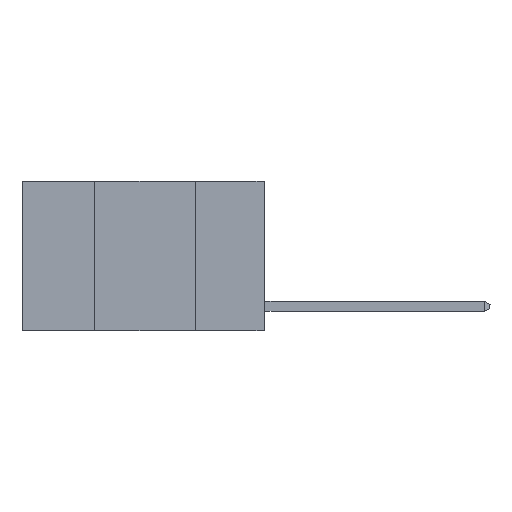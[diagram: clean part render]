
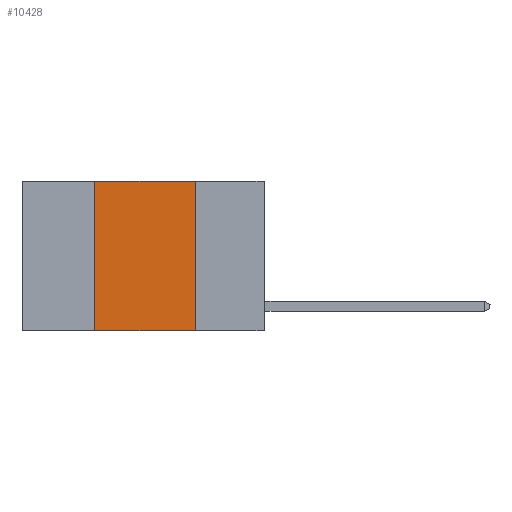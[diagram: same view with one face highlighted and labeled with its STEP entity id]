
A CAD part, left-side view. The second image highlights one B-rep face of the part: STEP entity #10428.
In plain terms, the highlighted planar face has unit normal (-1, 0, 0).
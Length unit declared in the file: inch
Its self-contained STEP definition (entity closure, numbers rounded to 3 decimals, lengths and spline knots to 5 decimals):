
#43 = VERTEX_POINT ( 'NONE', #5023 ) ;
#239 = VECTOR ( 'NONE', #8701, 39.37008 ) ;
#1864 = ORIENTED_EDGE ( 'NONE', *, *, #13951, .F. ) ;
#3717 = ORIENTED_EDGE ( 'NONE', *, *, #9097, .T. ) ;
#4014 = EDGE_CURVE ( 'NONE', #12205, #19481, #13334, .T. ) ;
#4199 = CARTESIAN_POINT ( 'NONE',  ( 0., 0.6, -0.37 ) ) ;
#4628 = CARTESIAN_POINT ( 'NONE',  ( 0., 0.42, 0. ) ) ;
#5023 = CARTESIAN_POINT ( 'NONE',  ( 0., 0.17, -0.37 ) ) ;
#5184 = DIRECTION ( 'NONE',  ( 0., 0., -1. ) ) ;
#5699 = VECTOR ( 'NONE', #17187, 39.37008 ) ;
#6202 = LINE ( 'NONE', #4199, #5699 ) ;
#6243 = CARTESIAN_POINT ( 'NONE',  ( 0., 0.42, 0. ) ) ;
#6359 = AXIS2_PLACEMENT_3D ( 'NONE', #9653, #20658, #11261 ) ;
#6722 = VERTEX_POINT ( 'NONE', #10295 ) ;
#6874 = EDGE_CURVE ( 'NONE', #6722, #12205, #18333, .T. ) ;
#7549 = VECTOR ( 'NONE', #5184, 39.37008 ) ;
#7879 = DIRECTION ( 'NONE',  ( 0., 0., 1. ) ) ;
#8475 = CARTESIAN_POINT ( 'NONE',  ( 0., 0.17, 0. ) ) ;
#8532 = CARTESIAN_POINT ( 'NONE',  ( 0., 0.17, 0. ) ) ;
#8701 = DIRECTION ( 'NONE',  ( 0., -1., 0. ) ) ;
#9097 = EDGE_CURVE ( 'NONE', #6722, #43, #6202, .T. ) ;
#9653 = CARTESIAN_POINT ( 'NONE',  ( 0., 0.6, 0. ) ) ;
#10295 = CARTESIAN_POINT ( 'NONE',  ( 0., 0.42, -0.37 ) ) ;
#10428 = ADVANCED_FACE ( 'NONE', ( #20076 ), #17589, .F. ) ;
#11129 = ORIENTED_EDGE ( 'NONE', *, *, #4014, .F. ) ;
#11261 = DIRECTION ( 'NONE',  ( 0., 0., -1. ) ) ;
#12205 = VERTEX_POINT ( 'NONE', #4628 ) ;
#13334 = LINE ( 'NONE', #16675, #239 ) ;
#13951 = EDGE_CURVE ( 'NONE', #19481, #43, #16112, .T. ) ;
#16112 = LINE ( 'NONE', #8475, #7549 ) ;
#16675 = CARTESIAN_POINT ( 'NONE',  ( 0., 0.6, 0. ) ) ;
#16718 = EDGE_LOOP ( 'NONE', ( #1864, #11129, #19512, #3717 ) ) ;
#17187 = DIRECTION ( 'NONE',  ( 0., -1., 0. ) ) ;
#17589 = PLANE ( 'NONE',  #6359 ) ;
#17847 = VECTOR ( 'NONE', #7879, 39.37008 ) ;
#18333 = LINE ( 'NONE', #6243, #17847 ) ;
#19481 = VERTEX_POINT ( 'NONE', #8532 ) ;
#19512 = ORIENTED_EDGE ( 'NONE', *, *, #6874, .F. ) ;
#20076 = FACE_OUTER_BOUND ( 'NONE', #16718, .T. ) ;
#20658 = DIRECTION ( 'NONE',  ( 1., 0., 0. ) ) ;
